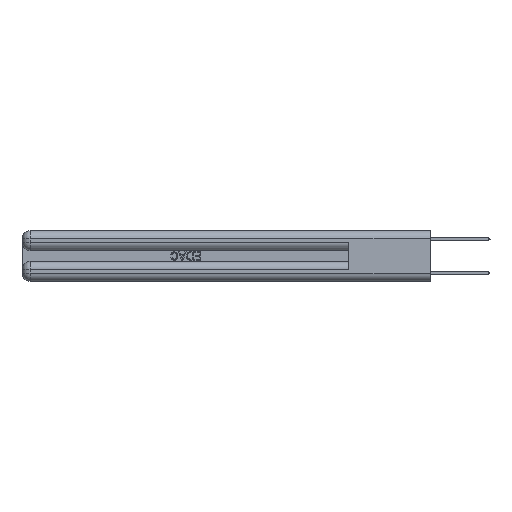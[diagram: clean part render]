
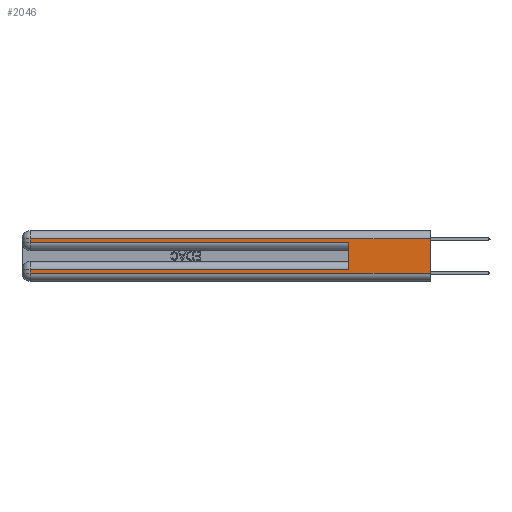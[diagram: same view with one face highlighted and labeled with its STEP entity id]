
A CAD part, left-side view. The second image highlights one B-rep face of the part: STEP entity #2046.
In plain terms, the highlighted planar face has unit normal (-1, 0, 0).
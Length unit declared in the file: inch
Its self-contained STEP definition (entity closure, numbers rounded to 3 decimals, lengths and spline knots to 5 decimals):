
#422 = EDGE_CURVE ( 'NONE', #17275, #19110, #22900, .T. ) ;
#594 = ORIENTED_EDGE ( 'NONE', *, *, #28268, .T. ) ;
#1196 = LINE ( 'NONE', #26614, #8371 ) ;
#1831 = CARTESIAN_POINT ( 'NONE',  ( 0., 0., 0.31 ) ) ;
#2046 = ADVANCED_FACE ( 'NONE', ( #7181 ), #24276, .F. ) ;
#2110 = AXIS2_PLACEMENT_3D ( 'NONE', #2995, #3615, #15380 ) ;
#2175 = CARTESIAN_POINT ( 'NONE',  ( 0., 0.6, 0.145 ) ) ;
#2995 = CARTESIAN_POINT ( 'NONE',  ( 0., 0., 0.37 ) ) ;
#3056 = ORIENTED_EDGE ( 'NONE', *, *, #14929, .T. ) ;
#3615 = DIRECTION ( 'NONE',  ( 1., 0., 0. ) ) ;
#4354 = DIRECTION ( 'NONE',  ( 0., -1., 0. ) ) ;
#4636 = LINE ( 'NONE', #6251, #16657 ) ;
#5204 = CARTESIAN_POINT ( 'NONE',  ( 0., 0.6, 0.285 ) ) ;
#5577 = CARTESIAN_POINT ( 'NONE',  ( 0., 0.6, 0.085 ) ) ;
#5745 = EDGE_CURVE ( 'NONE', #8147, #11045, #4636, .T. ) ;
#6251 = CARTESIAN_POINT ( 'NONE',  ( 0., 2.94, 0.37 ) ) ;
#7181 = FACE_OUTER_BOUND ( 'NONE', #23949, .T. ) ;
#7192 = LINE ( 'NONE', #14423, #10157 ) ;
#7227 = ORIENTED_EDGE ( 'NONE', *, *, #9247, .T. ) ;
#8147 = VERTEX_POINT ( 'NONE', #30092 ) ;
#8371 = VECTOR ( 'NONE', #24024, 39.37008 ) ;
#8781 = CARTESIAN_POINT ( 'NONE',  ( 0., 2.94, 0.06 ) ) ;
#8839 = ORIENTED_EDGE ( 'NONE', *, *, #422, .F. ) ;
#8872 = ORIENTED_EDGE ( 'NONE', *, *, #10153, .F. ) ;
#8964 = DIRECTION ( 'NONE',  ( 0., -1., 0. ) ) ;
#9069 = DIRECTION ( 'NONE',  ( 0., 0., -1. ) ) ;
#9247 = EDGE_CURVE ( 'NONE', #18903, #19110, #18555, .T. ) ;
#9678 = DIRECTION ( 'NONE',  ( 0., 0., -1. ) ) ;
#9919 = CARTESIAN_POINT ( 'NONE',  ( 0., 2.94, 0.085 ) ) ;
#10153 = EDGE_CURVE ( 'NONE', #22885, #10720, #11345, .T. ) ;
#10157 = VECTOR ( 'NONE', #16338, 39.37008 ) ;
#10505 = LINE ( 'NONE', #16824, #25825 ) ;
#10720 = VERTEX_POINT ( 'NONE', #5204 ) ;
#10951 = CARTESIAN_POINT ( 'NONE',  ( 0., 0., 0.37 ) ) ;
#11045 = VERTEX_POINT ( 'NONE', #19696 ) ;
#11345 = LINE ( 'NONE', #2175, #27108 ) ;
#14423 = CARTESIAN_POINT ( 'NONE',  ( 0., 0., 0.085 ) ) ;
#14427 = VECTOR ( 'NONE', #4354, 39.37008 ) ;
#14597 = EDGE_CURVE ( 'NONE', #22885, #30378, #7192, .T. ) ;
#14929 = EDGE_CURVE ( 'NONE', #30378, #18903, #10505, .T. ) ;
#15230 = ORIENTED_EDGE ( 'NONE', *, *, #26321, .T. ) ;
#15380 = DIRECTION ( 'NONE',  ( 0., 0., -1. ) ) ;
#16338 = DIRECTION ( 'NONE',  ( 0., 1., 0. ) ) ;
#16657 = VECTOR ( 'NONE', #9069, 39.37008 ) ;
#16824 = CARTESIAN_POINT ( 'NONE',  ( 0., 2.94, 0.37 ) ) ;
#17046 = CARTESIAN_POINT ( 'NONE',  ( 0., 0., 0.06 ) ) ;
#17275 = VERTEX_POINT ( 'NONE', #1831 ) ;
#17276 = ORIENTED_EDGE ( 'NONE', *, *, #14597, .T. ) ;
#18042 = VECTOR ( 'NONE', #23226, 39.37008 ) ;
#18555 = LINE ( 'NONE', #18734, #14427 ) ;
#18734 = CARTESIAN_POINT ( 'NONE',  ( 0., 0., 0.06 ) ) ;
#18903 = VERTEX_POINT ( 'NONE', #8781 ) ;
#19110 = VERTEX_POINT ( 'NONE', #17046 ) ;
#19386 = DIRECTION ( 'NONE',  ( 0., 0., 1. ) ) ;
#19696 = CARTESIAN_POINT ( 'NONE',  ( 0., 2.94, 0.285 ) ) ;
#22551 = ORIENTED_EDGE ( 'NONE', *, *, #5745, .T. ) ;
#22885 = VERTEX_POINT ( 'NONE', #5577 ) ;
#22900 = LINE ( 'NONE', #10951, #18042 ) ;
#23226 = DIRECTION ( 'NONE',  ( 0., 0., -1. ) ) ;
#23949 = EDGE_LOOP ( 'NONE', ( #8839, #15230, #22551, #594, #8872, #17276, #3056, #7227 ) ) ;
#24024 = DIRECTION ( 'NONE',  ( 0., 1., 0. ) ) ;
#24276 = PLANE ( 'NONE',  #2110 ) ;
#25011 = LINE ( 'NONE', #30934, #29925 ) ;
#25825 = VECTOR ( 'NONE', #9678, 39.37008 ) ;
#26321 = EDGE_CURVE ( 'NONE', #17275, #8147, #1196, .T. ) ;
#26614 = CARTESIAN_POINT ( 'NONE',  ( 0., 0., 0.31 ) ) ;
#27108 = VECTOR ( 'NONE', #19386, 39.37008 ) ;
#28268 = EDGE_CURVE ( 'NONE', #11045, #10720, #25011, .T. ) ;
#29925 = VECTOR ( 'NONE', #8964, 39.37008 ) ;
#30092 = CARTESIAN_POINT ( 'NONE',  ( 0., 2.94, 0.31 ) ) ;
#30378 = VERTEX_POINT ( 'NONE', #9919 ) ;
#30934 = CARTESIAN_POINT ( 'NONE',  ( 0., 0., 0.285 ) ) ;
